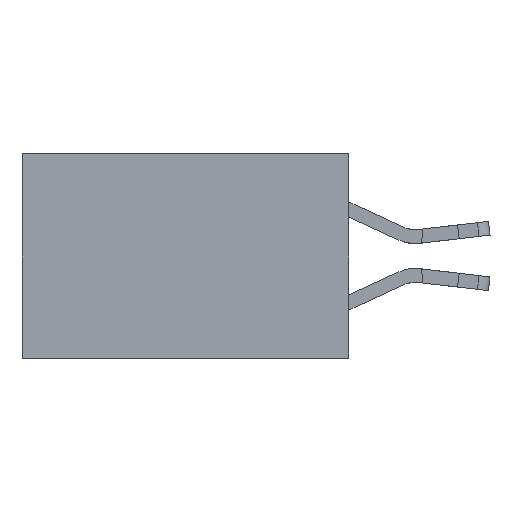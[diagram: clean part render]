
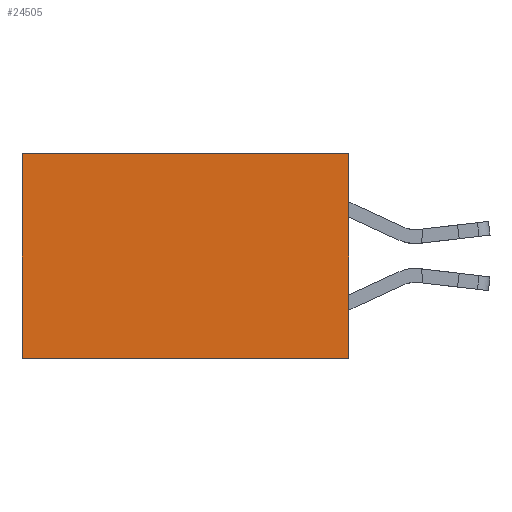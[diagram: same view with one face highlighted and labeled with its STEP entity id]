
A CAD part, left-side view. The second image highlights one B-rep face of the part: STEP entity #24505.
In plain terms, the highlighted planar face has unit normal (-1, 0, 0).
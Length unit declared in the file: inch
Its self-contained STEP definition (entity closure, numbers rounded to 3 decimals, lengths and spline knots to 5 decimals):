
#423 = VECTOR ( 'NONE', #5299, 39.37008 ) ;
#452 = EDGE_LOOP ( 'NONE', ( #13004, #18647, #28230, #26697 ) ) ;
#1311 = EDGE_CURVE ( 'NONE', #15032, #30717, #16078, .T. ) ;
#1803 = CARTESIAN_POINT ( 'NONE',  ( 0.277, 0., -0.37 ) ) ;
#3371 = VECTOR ( 'NONE', #17515, 39.37008 ) ;
#4248 = DIRECTION ( 'NONE',  ( 1., 0., 0. ) ) ;
#5299 = DIRECTION ( 'NONE',  ( 0., 1., 0. ) ) ;
#5565 = DIRECTION ( 'NONE',  ( 0., 0., -1. ) ) ;
#6856 = CARTESIAN_POINT ( 'NONE',  ( 0.277, 0., -0.37 ) ) ;
#6886 = LINE ( 'NONE', #12494, #423 ) ;
#9859 = LINE ( 'NONE', #12649, #3371 ) ;
#11486 = CARTESIAN_POINT ( 'NONE',  ( 0.277, 0.59, 0. ) ) ;
#11765 = EDGE_CURVE ( 'NONE', #24664, #29415, #9859, .T. ) ;
#12494 = CARTESIAN_POINT ( 'NONE',  ( 0.277, 0., 0. ) ) ;
#12649 = CARTESIAN_POINT ( 'NONE',  ( 0.277, 0., -0.37 ) ) ;
#13004 = ORIENTED_EDGE ( 'NONE', *, *, #1311, .T. ) ;
#13621 = AXIS2_PLACEMENT_3D ( 'NONE', #1803, #4248, #21137 ) ;
#15032 = VERTEX_POINT ( 'NONE', #11486 ) ;
#16078 = LINE ( 'NONE', #20869, #22411 ) ;
#16232 = EDGE_CURVE ( 'NONE', #29415, #30717, #18000, .T. ) ;
#16296 = PLANE ( 'NONE',  #13621 ) ;
#16704 = CARTESIAN_POINT ( 'NONE',  ( 0.277, 0., 0. ) ) ;
#17515 = DIRECTION ( 'NONE',  ( 0., 0., -1. ) ) ;
#18000 = LINE ( 'NONE', #6856, #23582 ) ;
#18647 = ORIENTED_EDGE ( 'NONE', *, *, #16232, .F. ) ;
#20869 = CARTESIAN_POINT ( 'NONE',  ( 0.277, 0.59, -0.37 ) ) ;
#21137 = DIRECTION ( 'NONE',  ( 0., 0., -1. ) ) ;
#22411 = VECTOR ( 'NONE', #5565, 39.37008 ) ;
#23582 = VECTOR ( 'NONE', #23659, 39.37008 ) ;
#23659 = DIRECTION ( 'NONE',  ( 0., 1., 0. ) ) ;
#24505 = ADVANCED_FACE ( 'NONE', ( #29643 ), #16296, .F. ) ;
#24664 = VERTEX_POINT ( 'NONE', #16704 ) ;
#26590 = CARTESIAN_POINT ( 'NONE',  ( 0.277, 0.59, -0.37 ) ) ;
#26697 = ORIENTED_EDGE ( 'NONE', *, *, #30073, .T. ) ;
#28230 = ORIENTED_EDGE ( 'NONE', *, *, #11765, .F. ) ;
#29175 = CARTESIAN_POINT ( 'NONE',  ( 0.277, 0., -0.37 ) ) ;
#29415 = VERTEX_POINT ( 'NONE', #29175 ) ;
#29643 = FACE_OUTER_BOUND ( 'NONE', #452, .T. ) ;
#30073 = EDGE_CURVE ( 'NONE', #24664, #15032, #6886, .T. ) ;
#30717 = VERTEX_POINT ( 'NONE', #26590 ) ;
